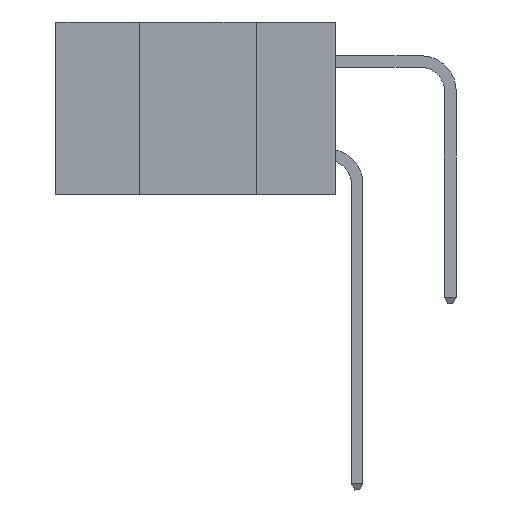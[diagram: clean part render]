
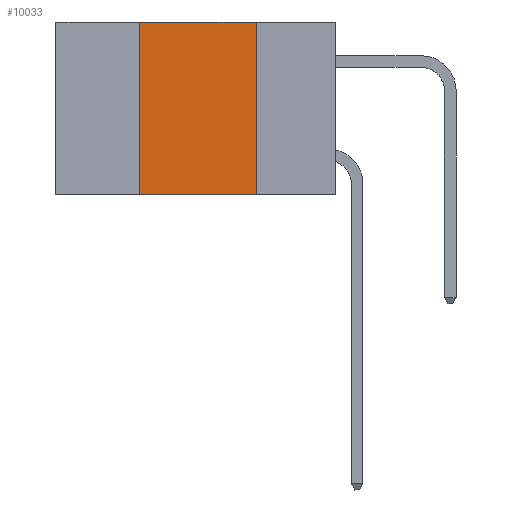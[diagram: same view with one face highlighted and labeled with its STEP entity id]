
A CAD part, left-side view. The second image highlights one B-rep face of the part: STEP entity #10033.
In plain terms, the highlighted planar face has unit normal (-1, 0, 0).
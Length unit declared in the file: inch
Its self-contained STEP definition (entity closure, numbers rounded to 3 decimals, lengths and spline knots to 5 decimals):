
#1777 = DIRECTION ( 'NONE',  ( 0., -1., 0. ) ) ;
#3216 = VECTOR ( 'NONE', #1777, 39.37008 ) ;
#4054 = CARTESIAN_POINT ( 'NONE',  ( 0., 0.6, 0. ) ) ;
#4356 = DIRECTION ( 'NONE',  ( 0., -1., 0. ) ) ;
#4615 = VERTEX_POINT ( 'NONE', #22026 ) ;
#5670 = ORIENTED_EDGE ( 'NONE', *, *, #24069, .T. ) ;
#5692 = ORIENTED_EDGE ( 'NONE', *, *, #7737, .F. ) ;
#5785 = VECTOR ( 'NONE', #19890, 39.37008 ) ;
#6272 = CARTESIAN_POINT ( 'NONE',  ( 0., 0.42, 0. ) ) ;
#6317 = LINE ( 'NONE', #15602, #8771 ) ;
#6378 = VERTEX_POINT ( 'NONE', #15410 ) ;
#7737 = EDGE_CURVE ( 'NONE', #25795, #4615, #23114, .T. ) ;
#8498 = LINE ( 'NONE', #26606, #3216 ) ;
#8771 = VECTOR ( 'NONE', #11095, 39.37008 ) ;
#9603 = EDGE_CURVE ( 'NONE', #6378, #25795, #17702, .T. ) ;
#10033 = ADVANCED_FACE ( 'NONE', ( #27465 ), #20563, .F. ) ;
#11060 = CARTESIAN_POINT ( 'NONE',  ( 0., 0.17, -0.37 ) ) ;
#11095 = DIRECTION ( 'NONE',  ( 0., 0., -1. ) ) ;
#12485 = EDGE_LOOP ( 'NONE', ( #25732, #5692, #21926, #5670 ) ) ;
#14991 = CARTESIAN_POINT ( 'NONE',  ( 0., 0.42, 0. ) ) ;
#15410 = CARTESIAN_POINT ( 'NONE',  ( 0., 0.42, -0.37 ) ) ;
#15602 = CARTESIAN_POINT ( 'NONE',  ( 0., 0.17, 0. ) ) ;
#16040 = CARTESIAN_POINT ( 'NONE',  ( 0., 0.6, 0. ) ) ;
#17702 = LINE ( 'NONE', #14991, #5785 ) ;
#17915 = VECTOR ( 'NONE', #4356, 39.37008 ) ;
#18592 = EDGE_CURVE ( 'NONE', #4615, #28299, #6317, .T. ) ;
#19890 = DIRECTION ( 'NONE',  ( 0., 0., 1. ) ) ;
#20563 = PLANE ( 'NONE',  #28376 ) ;
#21247 = DIRECTION ( 'NONE',  ( 0., 0., -1. ) ) ;
#21926 = ORIENTED_EDGE ( 'NONE', *, *, #9603, .F. ) ;
#22026 = CARTESIAN_POINT ( 'NONE',  ( 0., 0.17, 0. ) ) ;
#23114 = LINE ( 'NONE', #4054, #17915 ) ;
#24069 = EDGE_CURVE ( 'NONE', #6378, #28299, #8498, .T. ) ;
#25546 = DIRECTION ( 'NONE',  ( 1., 0., 0. ) ) ;
#25732 = ORIENTED_EDGE ( 'NONE', *, *, #18592, .F. ) ;
#25795 = VERTEX_POINT ( 'NONE', #6272 ) ;
#26606 = CARTESIAN_POINT ( 'NONE',  ( 0., 0.6, -0.37 ) ) ;
#27465 = FACE_OUTER_BOUND ( 'NONE', #12485, .T. ) ;
#28299 = VERTEX_POINT ( 'NONE', #11060 ) ;
#28376 = AXIS2_PLACEMENT_3D ( 'NONE', #16040, #25546, #21247 ) ;
